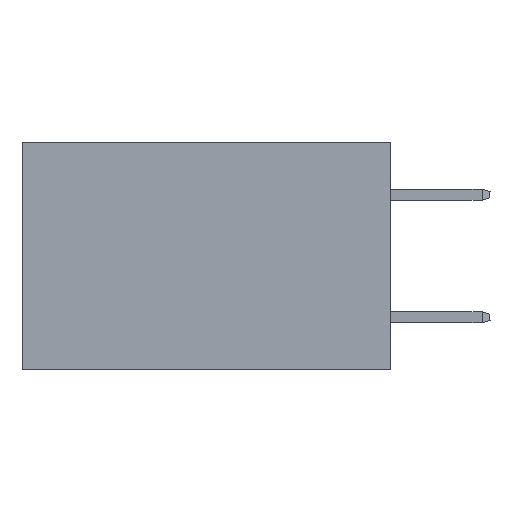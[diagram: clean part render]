
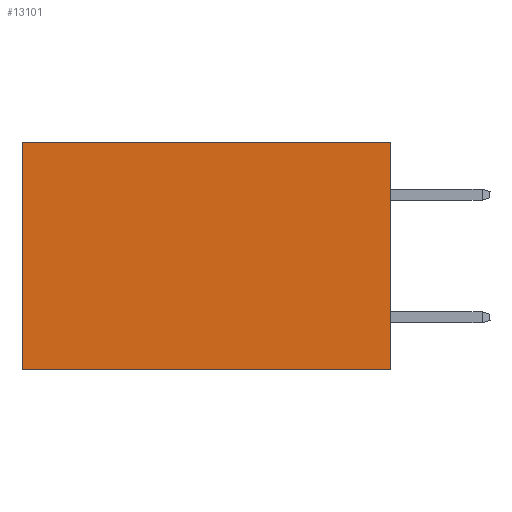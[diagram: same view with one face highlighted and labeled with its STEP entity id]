
A CAD part, left-side view. The second image highlights one B-rep face of the part: STEP entity #13101.
In plain terms, the highlighted planar face has unit normal (-1, 0, 0).
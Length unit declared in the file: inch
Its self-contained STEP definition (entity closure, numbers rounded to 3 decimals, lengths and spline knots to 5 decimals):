
#1821 = FACE_OUTER_BOUND ( 'NONE', #16947, .T. ) ;
#2643 = VERTEX_POINT ( 'NONE', #29102 ) ;
#3187 = CARTESIAN_POINT ( 'NONE',  ( 0.2875, 0.6, 0. ) ) ;
#4722 = LINE ( 'NONE', #11792, #5552 ) ;
#5015 = ORIENTED_EDGE ( 'NONE', *, *, #19965, .T. ) ;
#5552 = VECTOR ( 'NONE', #17094, 39.37008 ) ;
#6298 = DIRECTION ( 'NONE',  ( 0., 0., -1. ) ) ;
#7218 = DIRECTION ( 'NONE',  ( 0., 1., 0. ) ) ;
#7591 = DIRECTION ( 'NONE',  ( 0., 0., -1. ) ) ;
#7870 = CARTESIAN_POINT ( 'NONE',  ( 0.2875, 0., -0.37 ) ) ;
#8358 = ORIENTED_EDGE ( 'NONE', *, *, #31808, .F. ) ;
#9497 = LINE ( 'NONE', #9692, #23765 ) ;
#9692 = CARTESIAN_POINT ( 'NONE',  ( 0.2875, 0., -0.37 ) ) ;
#10535 = ORIENTED_EDGE ( 'NONE', *, *, #15331, .T. ) ;
#11792 = CARTESIAN_POINT ( 'NONE',  ( 0.2875, 0.6, 0. ) ) ;
#13080 = DIRECTION ( 'NONE',  ( 0., 1., 0. ) ) ;
#13101 = ADVANCED_FACE ( 'NONE', ( #1821 ), #22041, .F. ) ;
#15331 = EDGE_CURVE ( 'NONE', #23482, #32126, #15583, .T. ) ;
#15583 = LINE ( 'NONE', #18326, #18070 ) ;
#16947 = EDGE_LOOP ( 'NONE', ( #5015, #29839, #8358, #10535 ) ) ;
#17021 = AXIS2_PLACEMENT_3D ( 'NONE', #32668, #30206, #6298 ) ;
#17094 = DIRECTION ( 'NONE',  ( 0., 0., -1. ) ) ;
#18070 = VECTOR ( 'NONE', #7218, 39.37008 ) ;
#18326 = CARTESIAN_POINT ( 'NONE',  ( 0.2875, 0., 0. ) ) ;
#19965 = EDGE_CURVE ( 'NONE', #32126, #2643, #4722, .T. ) ;
#20667 = LINE ( 'NONE', #26056, #33204 ) ;
#22041 = PLANE ( 'NONE',  #17021 ) ;
#23482 = VERTEX_POINT ( 'NONE', #28466 ) ;
#23765 = VECTOR ( 'NONE', #13080, 39.37008 ) ;
#26056 = CARTESIAN_POINT ( 'NONE',  ( 0.2875, 0., 0. ) ) ;
#26301 = EDGE_CURVE ( 'NONE', #27176, #2643, #9497, .T. ) ;
#27176 = VERTEX_POINT ( 'NONE', #7870 ) ;
#28466 = CARTESIAN_POINT ( 'NONE',  ( 0.2875, 0., 0. ) ) ;
#29102 = CARTESIAN_POINT ( 'NONE',  ( 0.2875, 0.6, -0.37 ) ) ;
#29839 = ORIENTED_EDGE ( 'NONE', *, *, #26301, .F. ) ;
#30206 = DIRECTION ( 'NONE',  ( 1., 0., 0. ) ) ;
#31808 = EDGE_CURVE ( 'NONE', #23482, #27176, #20667, .T. ) ;
#32126 = VERTEX_POINT ( 'NONE', #3187 ) ;
#32668 = CARTESIAN_POINT ( 'NONE',  ( 0.2875, 0., 0. ) ) ;
#33204 = VECTOR ( 'NONE', #7591, 39.37008 ) ;
